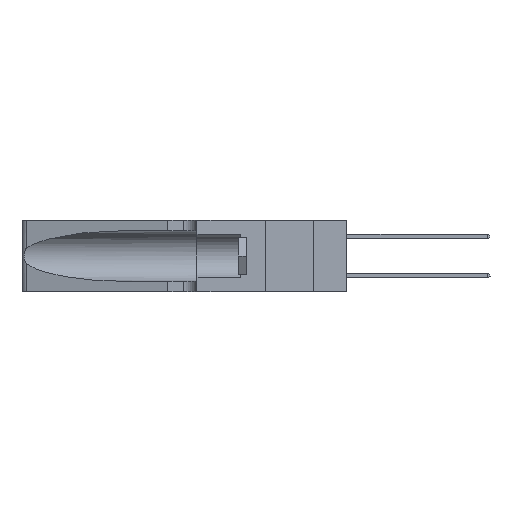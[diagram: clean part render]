
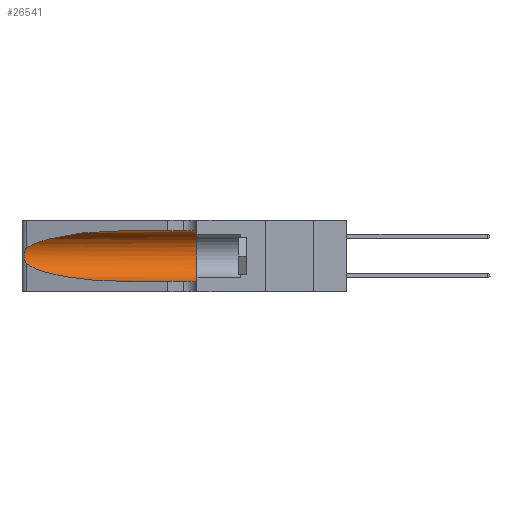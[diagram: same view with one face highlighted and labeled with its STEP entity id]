
A CAD part, left-side view. The second image highlights one B-rep face of the part: STEP entity #26541.
In plain terms, the highlighted cylindrical face has radius 3.308 mm (diameter 6.617 mm), a partial arc.
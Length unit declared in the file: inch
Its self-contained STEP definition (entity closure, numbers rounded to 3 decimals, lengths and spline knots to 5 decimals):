
#1297 = CARTESIAN_POINT ( 'NONE',  ( 0.1305, 0.35, 0.185 ) ) ;
#1511 = VERTEX_POINT ( 'NONE', #18060 ) ;
#2308 = CARTESIAN_POINT ( 'NONE',  ( 0.25487, 1.22718, 0.14631 ) ) ;
#2693 = CARTESIAN_POINT ( 'NONE',  ( 0.25487, 1.22718, 0.22369 ) ) ;
#4022 = CARTESIAN_POINT ( 'NONE',  ( 0.25854, 1.2359, 0.20912 ) ) ;
#4330 = CARTESIAN_POINT ( 'NONE',  ( 0.25639, 1.23186, 0.15144 ) ) ;
#4719 = EDGE_CURVE ( 'NONE', #29779, #25793, #17531, .T. ) ;
#6358 = DIRECTION ( 'NONE',  ( 0., 1., 0. ) ) ;
#6699 = CARTESIAN_POINT ( 'NONE',  ( 0.26018, 1.23835, 0.19895 ) ) ;
#6844 = CARTESIAN_POINT ( 'NONE',  ( 0.1305, 1.61858, 0.05475 ) ) ;
#9627 = CARTESIAN_POINT ( 'NONE',  ( 0.25639, 1.23184, 0.21858 ) ) ;
#9936 = EDGE_CURVE ( 'NONE', #29735, #29779, #14894, .T. ) ;
#10682 = ORIENTED_EDGE ( 'NONE', *, *, #10853, .F. ) ;
#10853 = EDGE_CURVE ( 'NONE', #24215, #11094, #30000, .T. ) ;
#11036 = CARTESIAN_POINT ( 'NONE',  ( 0.26075, 1.23896, 0.19203 ) ) ;
#11094 = VERTEX_POINT ( 'NONE', #15197 ) ;
#11690 = CARTESIAN_POINT ( 'NONE',  ( 0.26017, 1.23833, 0.17102 ) ) ;
#12893 = CARTESIAN_POINT ( 'NONE',  ( 0.25487, 1.22718, 0.14631 ) ) ;
#13604 = CARTESIAN_POINT ( 'NONE',  ( 0.25787, 1.23484, 0.2124 ) ) ;
#14540 = ORIENTED_EDGE ( 'NONE', *, *, #25504, .F. ) ;
#14695 = CARTESIAN_POINT ( 'NONE',  ( 0.18966, 0.96281, 0.31525 ) ) ;
#14736 = DIRECTION ( 'NONE',  ( 0., -1., 0. ) ) ;
#14894 = B_SPLINE_CURVE_WITH_KNOTS ( 'NONE', 3,
 ( #24716, #20733, #9627, #13604, #4022, #6699, #11036, #22304, #11690, #23867, #18720, #4330, #31122, #2308 ),
 .UNSPECIFIED., .F., .F.,
 ( 4, 2, 2, 2, 2, 2, 4 ),
 ( 0., 0.00027, 0.00053, 0.00107, 0.0016, 0.00187, 0.00214 ),
 .UNSPECIFIED. ) ;
#14936 = FACE_OUTER_BOUND ( 'NONE', #17201, .T. ) ;
#15197 = CARTESIAN_POINT ( 'NONE',  ( 0.1305, 0.35, 0.05475 ) ) ;
#15208 = CARTESIAN_POINT ( 'NONE',  ( 0.18966, 0.96281, 0.05475 ) ) ;
#15447 = LINE ( 'NONE', #6844, #21054 ) ;
#16528 = ORIENTED_EDGE ( 'NONE', *, *, #19065, .T. ) ;
#16621 =( BOUNDED_CURVE ( )  B_SPLINE_CURVE ( 3, ( #24229, #14695, #23836, #19302 ),
 .UNSPECIFIED., .F., .T. ) 
 B_SPLINE_CURVE_WITH_KNOTS ( ( 4, 4 ),
 ( 1.5708, 2.84003 ),
 .UNSPECIFIED. ) 
 CURVE ( )  GEOMETRIC_REPRESENTATION_ITEM ( )  RATIONAL_B_SPLINE_CURVE ( ( 1., 0.87, 0.87, 1. ) ) 
 REPRESENTATION_ITEM ( '' )  );
#17201 = EDGE_LOOP ( 'NONE', ( #16528, #23705, #26654, #22619, #10682, #14540 ) ) ;
#17464 = CARTESIAN_POINT ( 'NONE',  ( 0.2373, 1.15595, 0.08982 ) ) ;
#17531 =( BOUNDED_CURVE ( )  B_SPLINE_CURVE ( 3, ( #27356, #17464, #15208, #17557 ),
 .UNSPECIFIED., .F., .T. ) 
 B_SPLINE_CURVE_WITH_KNOTS ( ( 4, 4 ),
 ( 3.44316, 4.71239 ),
 .UNSPECIFIED. ) 
 CURVE ( )  GEOMETRIC_REPRESENTATION_ITEM ( )  RATIONAL_B_SPLINE_CURVE ( ( 1., 0.87, 0.87, 1. ) ) 
 REPRESENTATION_ITEM ( '' )  );
#17557 = CARTESIAN_POINT ( 'NONE',  ( 0.1305, 0.72297, 0.05475 ) ) ;
#18060 = CARTESIAN_POINT ( 'NONE',  ( 0.1305, 0.72297, 0.31525 ) ) ;
#18628 = DIRECTION ( 'NONE',  ( 0., 0., -1. ) ) ;
#18705 = DIRECTION ( 'NONE',  ( 0., -1., 0. ) ) ;
#18720 = CARTESIAN_POINT ( 'NONE',  ( 0.25789, 1.23486, 0.15765 ) ) ;
#19065 = EDGE_CURVE ( 'NONE', #1511, #29735, #16621, .T. ) ;
#19302 = CARTESIAN_POINT ( 'NONE',  ( 0.25487, 1.22718, 0.22369 ) ) ;
#20733 = CARTESIAN_POINT ( 'NONE',  ( 0.25555, 1.22994, 0.2215 ) ) ;
#21054 = VECTOR ( 'NONE', #18705, 39.37008 ) ;
#21333 = EDGE_CURVE ( 'NONE', #25793, #11094, #15447, .T. ) ;
#21370 = VECTOR ( 'NONE', #14736, 39.37008 ) ;
#22304 = CARTESIAN_POINT ( 'NONE',  ( 0.26075, 1.23896, 0.178 ) ) ;
#22619 = ORIENTED_EDGE ( 'NONE', *, *, #21333, .T. ) ;
#22946 = DIRECTION ( 'NONE',  ( 0., 0., 1. ) ) ;
#23275 = AXIS2_PLACEMENT_3D ( 'NONE', #26174, #28609, #18628 ) ;
#23705 = ORIENTED_EDGE ( 'NONE', *, *, #9936, .T. ) ;
#23836 = CARTESIAN_POINT ( 'NONE',  ( 0.2373, 1.15595, 0.28018 ) ) ;
#23867 = CARTESIAN_POINT ( 'NONE',  ( 0.25856, 1.23593, 0.16098 ) ) ;
#24215 = VERTEX_POINT ( 'NONE', #30992 ) ;
#24229 = CARTESIAN_POINT ( 'NONE',  ( 0.1305, 0.72297, 0.31525 ) ) ;
#24716 = CARTESIAN_POINT ( 'NONE',  ( 0.25487, 1.22718, 0.22369 ) ) ;
#25504 = EDGE_CURVE ( 'NONE', #1511, #24215, #27768, .T. ) ;
#25793 = VERTEX_POINT ( 'NONE', #27200 ) ;
#26069 = AXIS2_PLACEMENT_3D ( 'NONE', #1297, #6358, #22946 ) ;
#26174 = CARTESIAN_POINT ( 'NONE',  ( 0.1305, 1.61858, 0.185 ) ) ;
#26541 = ADVANCED_FACE ( 'NONE', ( #14936 ), #30355, .F. ) ;
#26654 = ORIENTED_EDGE ( 'NONE', *, *, #4719, .T. ) ;
#27200 = CARTESIAN_POINT ( 'NONE',  ( 0.1305, 0.72297, 0.05475 ) ) ;
#27356 = CARTESIAN_POINT ( 'NONE',  ( 0.25487, 1.22718, 0.14631 ) ) ;
#27768 = LINE ( 'NONE', #29320, #21370 ) ;
#28609 = DIRECTION ( 'NONE',  ( 0., -1., 0. ) ) ;
#29320 = CARTESIAN_POINT ( 'NONE',  ( 0.1305, 1.61858, 0.31525 ) ) ;
#29735 = VERTEX_POINT ( 'NONE', #2693 ) ;
#29779 = VERTEX_POINT ( 'NONE', #12893 ) ;
#30000 = CIRCLE ( 'NONE', #26069, 0.13025 ) ;
#30355 = CYLINDRICAL_SURFACE ( 'NONE', #23275, 0.13025 ) ;
#30992 = CARTESIAN_POINT ( 'NONE',  ( 0.1305, 0.35, 0.31525 ) ) ;
#31122 = CARTESIAN_POINT ( 'NONE',  ( 0.25555, 1.22993, 0.14849 ) ) ;
